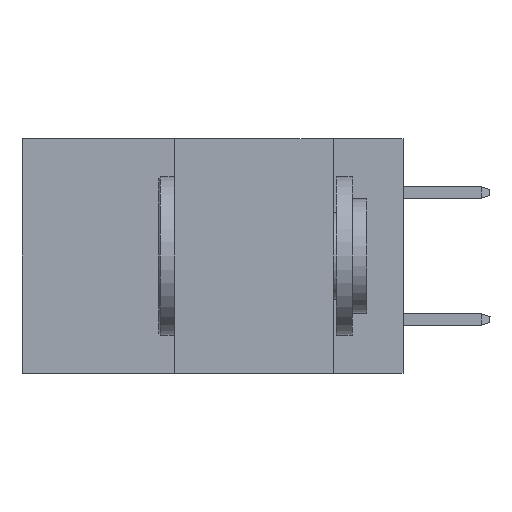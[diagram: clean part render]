
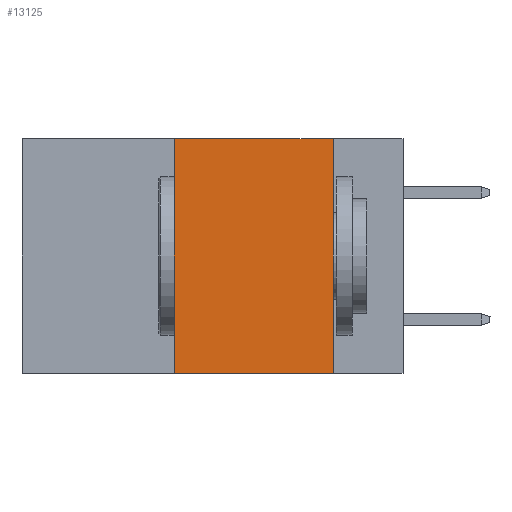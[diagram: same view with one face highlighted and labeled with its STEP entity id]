
A CAD part, left-side view. The second image highlights one B-rep face of the part: STEP entity #13125.
In plain terms, the highlighted planar face has unit normal (-1, 0, 0).
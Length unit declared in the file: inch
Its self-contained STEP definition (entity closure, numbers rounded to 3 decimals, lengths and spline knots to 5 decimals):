
#826 = CARTESIAN_POINT ( 'NONE',  ( 0., 0.11, 0. ) ) ;
#1325 = VECTOR ( 'NONE', #27918, 39.37008 ) ;
#2823 = CARTESIAN_POINT ( 'NONE',  ( 0., 0.6, 0. ) ) ;
#3362 = EDGE_CURVE ( 'NONE', #3760, #7612, #16799, .T. ) ;
#3760 = VERTEX_POINT ( 'NONE', #5005 ) ;
#4051 = ORIENTED_EDGE ( 'NONE', *, *, #6881, .T. ) ;
#5005 = CARTESIAN_POINT ( 'NONE',  ( 0., 0.36, -0.37 ) ) ;
#6881 = EDGE_CURVE ( 'NONE', #3760, #27539, #17579, .T. ) ;
#7612 = VERTEX_POINT ( 'NONE', #8971 ) ;
#8318 = EDGE_CURVE ( 'NONE', #7612, #32156, #12607, .T. ) ;
#8971 = CARTESIAN_POINT ( 'NONE',  ( 0., 0.36, 0. ) ) ;
#9904 = EDGE_CURVE ( 'NONE', #32156, #27539, #28240, .T. ) ;
#11279 = FACE_OUTER_BOUND ( 'NONE', #23927, .T. ) ;
#12155 = VECTOR ( 'NONE', #16446, 39.37008 ) ;
#12607 = LINE ( 'NONE', #2823, #17089 ) ;
#13125 = ADVANCED_FACE ( 'NONE', ( #11279 ), #21010, .F. ) ;
#13797 = DIRECTION ( 'NONE',  ( 0., 0., -1. ) ) ;
#14819 = CARTESIAN_POINT ( 'NONE',  ( 0., 0.11, 0. ) ) ;
#15439 = DIRECTION ( 'NONE',  ( 0., -1., 0. ) ) ;
#16446 = DIRECTION ( 'NONE',  ( 0., 0., 1. ) ) ;
#16799 = LINE ( 'NONE', #24491, #12155 ) ;
#17089 = VECTOR ( 'NONE', #15439, 39.37008 ) ;
#17579 = LINE ( 'NONE', #22623, #27473 ) ;
#18042 = AXIS2_PLACEMENT_3D ( 'NONE', #21531, #28746, #13797 ) ;
#18850 = ORIENTED_EDGE ( 'NONE', *, *, #3362, .F. ) ;
#21010 = PLANE ( 'NONE',  #18042 ) ;
#21531 = CARTESIAN_POINT ( 'NONE',  ( 0., 0.6, 0. ) ) ;
#21923 = ORIENTED_EDGE ( 'NONE', *, *, #9904, .F. ) ;
#22274 = ORIENTED_EDGE ( 'NONE', *, *, #8318, .F. ) ;
#22623 = CARTESIAN_POINT ( 'NONE',  ( 0., 0.6, -0.37 ) ) ;
#23927 = EDGE_LOOP ( 'NONE', ( #21923, #22274, #18850, #4051 ) ) ;
#24491 = CARTESIAN_POINT ( 'NONE',  ( 0., 0.36, 0. ) ) ;
#27473 = VECTOR ( 'NONE', #30506, 39.37008 ) ;
#27539 = VERTEX_POINT ( 'NONE', #28246 ) ;
#27918 = DIRECTION ( 'NONE',  ( 0., 0., -1. ) ) ;
#28240 = LINE ( 'NONE', #14819, #1325 ) ;
#28246 = CARTESIAN_POINT ( 'NONE',  ( 0., 0.11, -0.37 ) ) ;
#28746 = DIRECTION ( 'NONE',  ( 1., 0., 0. ) ) ;
#30506 = DIRECTION ( 'NONE',  ( 0., -1., 0. ) ) ;
#32156 = VERTEX_POINT ( 'NONE', #826 ) ;
